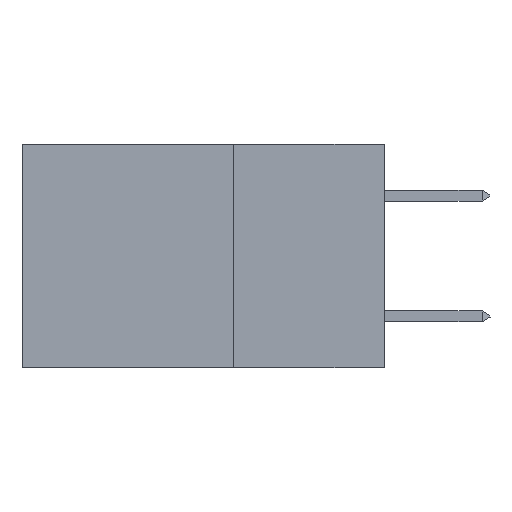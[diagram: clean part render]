
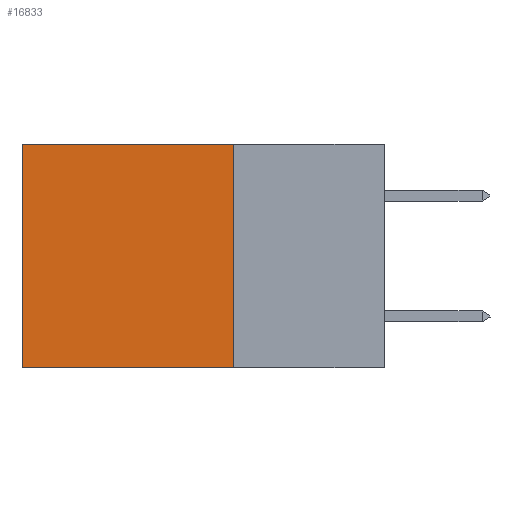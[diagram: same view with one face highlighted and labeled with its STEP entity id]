
A CAD part, left-side view. The second image highlights one B-rep face of the part: STEP entity #16833.
In plain terms, the highlighted planar face has unit normal (-1, 0, 0).
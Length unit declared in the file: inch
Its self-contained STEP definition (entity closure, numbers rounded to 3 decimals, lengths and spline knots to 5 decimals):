
#404 = VERTEX_POINT ( 'NONE', #7571 ) ;
#650 = EDGE_CURVE ( 'NONE', #404, #4326, #6103, .T. ) ;
#680 = LINE ( 'NONE', #14628, #8365 ) ;
#1629 = PLANE ( 'NONE',  #3642 ) ;
#2306 = ORIENTED_EDGE ( 'NONE', *, *, #16464, .T. ) ;
#3183 = DIRECTION ( 'NONE',  ( 1., 0., 0. ) ) ;
#3370 = CARTESIAN_POINT ( 'NONE',  ( 0.2875, 0.25, 0. ) ) ;
#3642 = AXIS2_PLACEMENT_3D ( 'NONE', #16611, #3183, #12514 ) ;
#4289 = VERTEX_POINT ( 'NONE', #14825 ) ;
#4326 = VERTEX_POINT ( 'NONE', #12616 ) ;
#5323 = VECTOR ( 'NONE', #12584, 39.37008 ) ;
#5819 = DIRECTION ( 'NONE',  ( 0., 1., 0. ) ) ;
#5826 = CARTESIAN_POINT ( 'NONE',  ( 0.2875, 0.25, 0. ) ) ;
#6103 = LINE ( 'NONE', #9030, #7377 ) ;
#7377 = VECTOR ( 'NONE', #7564, 39.37008 ) ;
#7564 = DIRECTION ( 'NONE',  ( 0., 1., 0. ) ) ;
#7571 = CARTESIAN_POINT ( 'NONE',  ( 0.2875, 0.25, -0.37 ) ) ;
#8365 = VECTOR ( 'NONE', #12534, 39.37008 ) ;
#8766 = EDGE_CURVE ( 'NONE', #11963, #404, #12071, .T. ) ;
#9030 = CARTESIAN_POINT ( 'NONE',  ( 0.2875, 0.25, -0.37 ) ) ;
#9470 = LINE ( 'NONE', #3370, #9892 ) ;
#9892 = VECTOR ( 'NONE', #5819, 39.37008 ) ;
#10006 = CARTESIAN_POINT ( 'NONE',  ( 0.2875, 0.25, 0. ) ) ;
#11649 = ORIENTED_EDGE ( 'NONE', *, *, #8766, .F. ) ;
#11963 = VERTEX_POINT ( 'NONE', #10006 ) ;
#12071 = LINE ( 'NONE', #5826, #5323 ) ;
#12514 = DIRECTION ( 'NONE',  ( 0., 0., -1. ) ) ;
#12534 = DIRECTION ( 'NONE',  ( 0., 0., -1. ) ) ;
#12584 = DIRECTION ( 'NONE',  ( 0., 0., -1. ) ) ;
#12616 = CARTESIAN_POINT ( 'NONE',  ( 0.2875, 0.6, -0.37 ) ) ;
#14289 = FACE_OUTER_BOUND ( 'NONE', #16676, .T. ) ;
#14367 = ORIENTED_EDGE ( 'NONE', *, *, #15845, .T. ) ;
#14628 = CARTESIAN_POINT ( 'NONE',  ( 0.2875, 0.6, 0. ) ) ;
#14825 = CARTESIAN_POINT ( 'NONE',  ( 0.2875, 0.6, 0. ) ) ;
#14885 = ORIENTED_EDGE ( 'NONE', *, *, #650, .F. ) ;
#15845 = EDGE_CURVE ( 'NONE', #4289, #4326, #680, .T. ) ;
#16464 = EDGE_CURVE ( 'NONE', #11963, #4289, #9470, .T. ) ;
#16611 = CARTESIAN_POINT ( 'NONE',  ( 0.2875, 0.25, 0. ) ) ;
#16676 = EDGE_LOOP ( 'NONE', ( #14367, #14885, #11649, #2306 ) ) ;
#16833 = ADVANCED_FACE ( 'NONE', ( #14289 ), #1629, .F. ) ;
